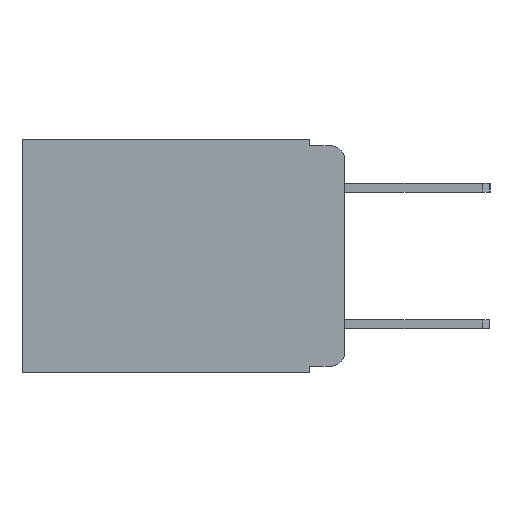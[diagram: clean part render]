
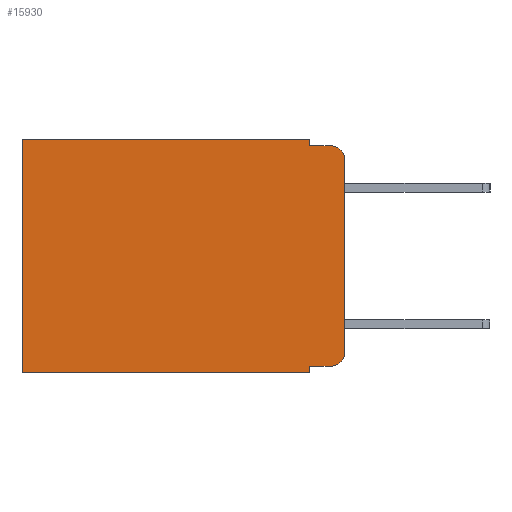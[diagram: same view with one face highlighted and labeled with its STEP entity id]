
A CAD part, left-side view. The second image highlights one B-rep face of the part: STEP entity #15930.
In plain terms, the highlighted planar face has unit normal (-1, 0, 0).
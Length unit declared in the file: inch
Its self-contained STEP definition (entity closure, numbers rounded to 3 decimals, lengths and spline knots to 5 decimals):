
#427 = DIRECTION ( 'NONE',  ( 0., 0., -1. ) ) ;
#1066 = DIRECTION ( 'NONE',  ( 0., 0., -1. ) ) ;
#1215 = DIRECTION ( 'NONE',  ( -1., 0., 0. ) ) ;
#1672 = VERTEX_POINT ( 'NONE', #2619 ) ;
#1720 = ORIENTED_EDGE ( 'NONE', *, *, #3691, .F. ) ;
#1758 = VERTEX_POINT ( 'NONE', #3065 ) ;
#2069 = LINE ( 'NONE', #11037, #15040 ) ;
#2485 = VECTOR ( 'NONE', #12074, 39.37008 ) ;
#2516 = VERTEX_POINT ( 'NONE', #9560 ) ;
#2543 = LINE ( 'NONE', #10652, #9653 ) ;
#2619 = CARTESIAN_POINT ( 'NONE',  ( 0.298, 0.02, -0.333 ) ) ;
#2683 = CARTESIAN_POINT ( 'NONE',  ( 0.298, 0.051, 0. ) ) ;
#3065 = CARTESIAN_POINT ( 'NONE',  ( 0.298, 0.473, -0.343 ) ) ;
#3144 = EDGE_CURVE ( 'NONE', #6924, #1758, #14553, .T. ) ;
#3228 = EDGE_CURVE ( 'NONE', #11812, #7847, #2543, .T. ) ;
#3250 = ORIENTED_EDGE ( 'NONE', *, *, #3228, .T. ) ;
#3259 = EDGE_CURVE ( 'NONE', #7281, #4387, #2069, .T. ) ;
#3355 = EDGE_CURVE ( 'NONE', #2516, #1672, #16498, .T. ) ;
#3528 = CARTESIAN_POINT ( 'NONE',  ( 0.298, 0.473, 0. ) ) ;
#3622 = EDGE_CURVE ( 'NONE', #7281, #11794, #4613, .T. ) ;
#3677 = ORIENTED_EDGE ( 'NONE', *, *, #4197, .F. ) ;
#3691 = EDGE_CURVE ( 'NONE', #2516, #6924, #10987, .T. ) ;
#3733 = DIRECTION ( 'NONE',  ( -1., 0., 0. ) ) ;
#3903 = ORIENTED_EDGE ( 'NONE', *, *, #3259, .F. ) ;
#3937 = VECTOR ( 'NONE', #4938, 39.37008 ) ;
#4140 = VECTOR ( 'NONE', #16686, 39.37008 ) ;
#4195 = EDGE_CURVE ( 'NONE', #7847, #1758, #10007, .T. ) ;
#4197 = EDGE_CURVE ( 'NONE', #6416, #11794, #12787, .T. ) ;
#4219 = EDGE_CURVE ( 'NONE', #11812, #6416, #15322, .T. ) ;
#4387 = VERTEX_POINT ( 'NONE', #11424 ) ;
#4600 = EDGE_CURVE ( 'NONE', #1672, #4387, #12902, .T. ) ;
#4613 = CIRCLE ( 'NONE', #5175, 0.02 ) ;
#4882 = DIRECTION ( 'NONE',  ( 0., -1., 0. ) ) ;
#4938 = DIRECTION ( 'NONE',  ( 0., 1., 0. ) ) ;
#5175 = AXIS2_PLACEMENT_3D ( 'NONE', #8257, #1215, #11039 ) ;
#5461 = VECTOR ( 'NONE', #1066, 39.37008 ) ;
#5557 = DIRECTION ( 'NONE',  ( 0., 1., 0. ) ) ;
#5651 = CARTESIAN_POINT ( 'NONE',  ( 0.298, 0.02, -0.01 ) ) ;
#6416 = VERTEX_POINT ( 'NONE', #6612 ) ;
#6612 = CARTESIAN_POINT ( 'NONE',  ( 0.298, 0.051, -0.01 ) ) ;
#6640 = CARTESIAN_POINT ( 'NONE',  ( 0.298, 0., -0.03 ) ) ;
#6827 = CARTESIAN_POINT ( 'NONE',  ( 0.298, 0.051, -0.333 ) ) ;
#6848 = CARTESIAN_POINT ( 'NONE',  ( 0.298, 0., -0.343 ) ) ;
#6924 = VERTEX_POINT ( 'NONE', #10703 ) ;
#7117 = CARTESIAN_POINT ( 'NONE',  ( 0.298, 0.051, -0.01 ) ) ;
#7281 = VERTEX_POINT ( 'NONE', #6640 ) ;
#7420 = PLANE ( 'NONE',  #13937 ) ;
#7847 = VERTEX_POINT ( 'NONE', #3528 ) ;
#8257 = CARTESIAN_POINT ( 'NONE',  ( 0.298, 0.02, -0.03 ) ) ;
#8677 = ORIENTED_EDGE ( 'NONE', *, *, #3144, .F. ) ;
#8834 = DIRECTION ( 'NONE',  ( 0., 0., -1. ) ) ;
#9263 = ORIENTED_EDGE ( 'NONE', *, *, #4195, .T. ) ;
#9560 = CARTESIAN_POINT ( 'NONE',  ( 0.298, 0.051, -0.333 ) ) ;
#9603 = VECTOR ( 'NONE', #14338, 39.37008 ) ;
#9653 = VECTOR ( 'NONE', #5557, 39.37008 ) ;
#9726 = CARTESIAN_POINT ( 'NONE',  ( 0.298, 0.473, 0. ) ) ;
#9833 = CARTESIAN_POINT ( 'NONE',  ( 0.298, 0.051, 0. ) ) ;
#9981 = DIRECTION ( 'NONE',  ( 0., 0., -1. ) ) ;
#10007 = LINE ( 'NONE', #9726, #9603 ) ;
#10652 = CARTESIAN_POINT ( 'NONE',  ( 0.298, 0., 0. ) ) ;
#10703 = CARTESIAN_POINT ( 'NONE',  ( 0.298, 0.051, -0.343 ) ) ;
#10777 = AXIS2_PLACEMENT_3D ( 'NONE', #11838, #3733, #427 ) ;
#10959 = ORIENTED_EDGE ( 'NONE', *, *, #3355, .T. ) ;
#10987 = LINE ( 'NONE', #2683, #4140 ) ;
#11037 = CARTESIAN_POINT ( 'NONE',  ( 0.298, 0., 0. ) ) ;
#11039 = DIRECTION ( 'NONE',  ( 0., 0., -1. ) ) ;
#11424 = CARTESIAN_POINT ( 'NONE',  ( 0.298, 0., -0.313 ) ) ;
#11794 = VERTEX_POINT ( 'NONE', #5651 ) ;
#11812 = VERTEX_POINT ( 'NONE', #9833 ) ;
#11838 = CARTESIAN_POINT ( 'NONE',  ( 0.298, 0.02, -0.313 ) ) ;
#11925 = ORIENTED_EDGE ( 'NONE', *, *, #3622, .T. ) ;
#12074 = DIRECTION ( 'NONE',  ( 0., -1., 0. ) ) ;
#12787 = LINE ( 'NONE', #7117, #2485 ) ;
#12902 = CIRCLE ( 'NONE', #10777, 0.02 ) ;
#13213 = CARTESIAN_POINT ( 'NONE',  ( 0.298, 0.051, 0. ) ) ;
#13703 = VECTOR ( 'NONE', #4882, 39.37008 ) ;
#13709 = EDGE_LOOP ( 'NONE', ( #3903, #11925, #3677, #14191, #3250, #9263, #8677, #1720, #10959, #15492 ) ) ;
#13937 = AXIS2_PLACEMENT_3D ( 'NONE', #14682, #15717, #8834 ) ;
#14191 = ORIENTED_EDGE ( 'NONE', *, *, #4219, .F. ) ;
#14338 = DIRECTION ( 'NONE',  ( 0., 0., -1. ) ) ;
#14553 = LINE ( 'NONE', #6848, #3937 ) ;
#14682 = CARTESIAN_POINT ( 'NONE',  ( 0.298, 0., 0. ) ) ;
#14819 = FACE_OUTER_BOUND ( 'NONE', #13709, .T. ) ;
#15040 = VECTOR ( 'NONE', #9981, 39.37008 ) ;
#15322 = LINE ( 'NONE', #13213, #5461 ) ;
#15492 = ORIENTED_EDGE ( 'NONE', *, *, #4600, .T. ) ;
#15717 = DIRECTION ( 'NONE',  ( 1., 0., 0. ) ) ;
#15930 = ADVANCED_FACE ( 'NONE', ( #14819 ), #7420, .F. ) ;
#16498 = LINE ( 'NONE', #6827, #13703 ) ;
#16686 = DIRECTION ( 'NONE',  ( 0., 0., -1. ) ) ;
